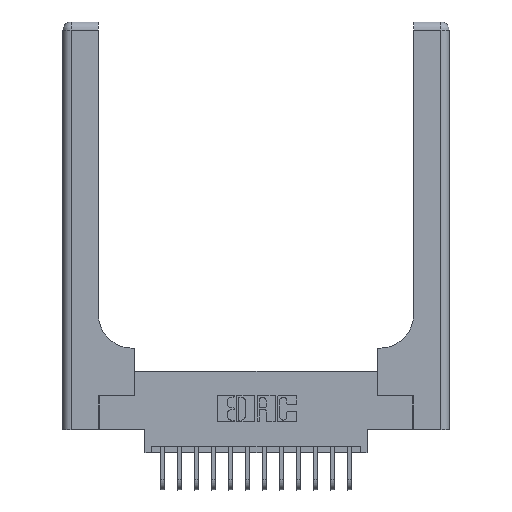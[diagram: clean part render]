
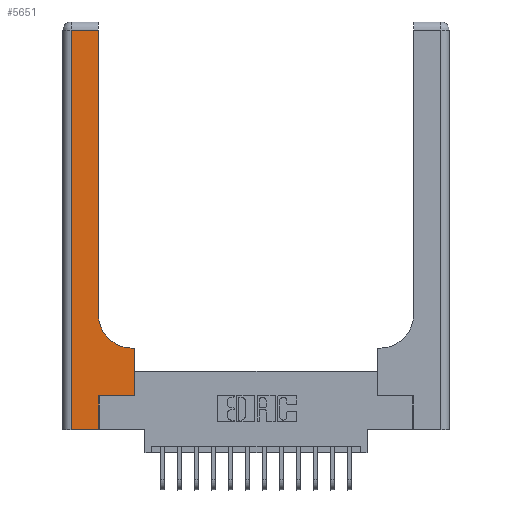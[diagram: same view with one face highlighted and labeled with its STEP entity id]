
A CAD part, top view. The second image highlights one B-rep face of the part: STEP entity #5651.
In plain terms, the highlighted planar face has unit normal (0, 0, 1).
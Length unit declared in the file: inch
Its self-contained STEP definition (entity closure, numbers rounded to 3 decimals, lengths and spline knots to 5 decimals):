
#55 = DIRECTION ( 'NONE',  ( 0., 1., 0. ) ) ;
#340 = EDGE_CURVE ( 'NONE', #1381, #548, #7350, .T. ) ;
#395 = FACE_OUTER_BOUND ( 'NONE', #15063, .T. ) ;
#422 = VERTEX_POINT ( 'NONE', #14021 ) ;
#503 = CARTESIAN_POINT ( 'NONE',  ( 0.528, 0.25, 0.37 ) ) ;
#518 = DIRECTION ( 'NONE',  ( 0., 0., -1. ) ) ;
#548 = VERTEX_POINT ( 'NONE', #11498 ) ;
#1215 = VECTOR ( 'NONE', #4240, 39.37008 ) ;
#1381 = VERTEX_POINT ( 'NONE', #14189 ) ;
#1453 = LINE ( 'NONE', #6443, #2290 ) ;
#1654 = ORIENTED_EDGE ( 'NONE', *, *, #1774, .T. ) ;
#1774 = EDGE_CURVE ( 'NONE', #3739, #4242, #1453, .T. ) ;
#1824 = DIRECTION ( 'NONE',  ( 0., 1., 0. ) ) ;
#2117 = LINE ( 'NONE', #503, #8754 ) ;
#2120 = ORIENTED_EDGE ( 'NONE', *, *, #7879, .T. ) ;
#2214 = LINE ( 'NONE', #14108, #15675 ) ;
#2290 = VECTOR ( 'NONE', #13499, 39.37008 ) ;
#2373 = LINE ( 'NONE', #11804, #15837 ) ;
#2389 = DIRECTION ( 'NONE',  ( 0., 1., 0. ) ) ;
#2402 = ORIENTED_EDGE ( 'NONE', *, *, #3684, .T. ) ;
#2925 = CARTESIAN_POINT ( 'NONE',  ( 0.528, 0.25, 0.37 ) ) ;
#3399 = VECTOR ( 'NONE', #15472, 39.37008 ) ;
#3684 = EDGE_CURVE ( 'NONE', #4242, #1381, #2117, .T. ) ;
#3739 = VERTEX_POINT ( 'NONE', #5965 ) ;
#4028 = CARTESIAN_POINT ( 'NONE',  ( 0.06, 2.94, 0.37 ) ) ;
#4240 = DIRECTION ( 'NONE',  ( 1., 0., 0. ) ) ;
#4242 = VERTEX_POINT ( 'NONE', #2925 ) ;
#4299 = CIRCLE ( 'NONE', #7024, 0.25 ) ;
#4398 = LINE ( 'NONE', #12008, #1215 ) ;
#4882 = CARTESIAN_POINT ( 'NONE',  ( 0.51, 0.85, 0.37 ) ) ;
#4971 = VERTEX_POINT ( 'NONE', #9056 ) ;
#5651 = ADVANCED_FACE ( 'NONE', ( #395 ), #12270, .F. ) ;
#5926 = VERTEX_POINT ( 'NONE', #7805 ) ;
#5965 = CARTESIAN_POINT ( 'NONE',  ( 0.265, 0.25, 0.37 ) ) ;
#6222 = DIRECTION ( 'NONE',  ( 1., 0., 0. ) ) ;
#6296 = ORIENTED_EDGE ( 'NONE', *, *, #10732, .T. ) ;
#6400 = VECTOR ( 'NONE', #8254, 39.37008 ) ;
#6443 = CARTESIAN_POINT ( 'NONE',  ( 0.265, 0.25, 0.37 ) ) ;
#6940 = CARTESIAN_POINT ( 'NONE',  ( 0., 2.94, 0.37 ) ) ;
#7024 = AXIS2_PLACEMENT_3D ( 'NONE', #4882, #13938, #6222 ) ;
#7350 = LINE ( 'NONE', #16015, #3399 ) ;
#7425 = ORIENTED_EDGE ( 'NONE', *, *, #11349, .T. ) ;
#7805 = CARTESIAN_POINT ( 'NONE',  ( 0.26, 0.85, 0.37 ) ) ;
#7879 = EDGE_CURVE ( 'NONE', #548, #5926, #4299, .T. ) ;
#8254 = DIRECTION ( 'NONE',  ( -1., 0., 0. ) ) ;
#8291 = CARTESIAN_POINT ( 'NONE',  ( 0.265, 0., 0.37 ) ) ;
#8470 = CARTESIAN_POINT ( 'NONE',  ( 0., 3., 0.37 ) ) ;
#8754 = VECTOR ( 'NONE', #1824, 39.37008 ) ;
#8766 = EDGE_CURVE ( 'NONE', #13071, #422, #10026, .T. ) ;
#9056 = CARTESIAN_POINT ( 'NONE',  ( 0.26, 2.94, 0.37 ) ) ;
#9779 = DIRECTION ( 'NONE',  ( -1., 0., 0. ) ) ;
#9852 = LINE ( 'NONE', #6940, #6400 ) ;
#10026 = LINE ( 'NONE', #14906, #12209 ) ;
#10732 = EDGE_CURVE ( 'NONE', #13164, #3739, #2214, .T. ) ;
#10830 = ORIENTED_EDGE ( 'NONE', *, *, #15857, .T. ) ;
#11349 = EDGE_CURVE ( 'NONE', #4971, #13071, #9852, .T. ) ;
#11498 = CARTESIAN_POINT ( 'NONE',  ( 0.51, 0.6, 0.37 ) ) ;
#11804 = CARTESIAN_POINT ( 'NONE',  ( 0.26, 3., 0.37 ) ) ;
#11869 = EDGE_CURVE ( 'NONE', #5926, #4971, #2373, .T. ) ;
#12008 = CARTESIAN_POINT ( 'NONE',  ( 0., 0., 0.37 ) ) ;
#12209 = VECTOR ( 'NONE', #16204, 39.37008 ) ;
#12270 = PLANE ( 'NONE',  #13577 ) ;
#13071 = VERTEX_POINT ( 'NONE', #4028 ) ;
#13164 = VERTEX_POINT ( 'NONE', #8291 ) ;
#13499 = DIRECTION ( 'NONE',  ( 1., 0., 0. ) ) ;
#13577 = AXIS2_PLACEMENT_3D ( 'NONE', #8470, #518, #9779 ) ;
#13938 = DIRECTION ( 'NONE',  ( 0., 0., -1. ) ) ;
#14021 = CARTESIAN_POINT ( 'NONE',  ( 0.06, 0., 0.37 ) ) ;
#14108 = CARTESIAN_POINT ( 'NONE',  ( 0.265, 0., 0.37 ) ) ;
#14189 = CARTESIAN_POINT ( 'NONE',  ( 0.528, 0.6, 0.37 ) ) ;
#14647 = ORIENTED_EDGE ( 'NONE', *, *, #11869, .T. ) ;
#14906 = CARTESIAN_POINT ( 'NONE',  ( 0.06, 3., 0.37 ) ) ;
#15063 = EDGE_LOOP ( 'NONE', ( #14647, #7425, #15755, #10830, #6296, #1654, #2402, #16491, #2120 ) ) ;
#15472 = DIRECTION ( 'NONE',  ( -1., 0., 0. ) ) ;
#15675 = VECTOR ( 'NONE', #2389, 39.37008 ) ;
#15755 = ORIENTED_EDGE ( 'NONE', *, *, #8766, .T. ) ;
#15837 = VECTOR ( 'NONE', #55, 39.37008 ) ;
#15857 = EDGE_CURVE ( 'NONE', #422, #13164, #4398, .T. ) ;
#16015 = CARTESIAN_POINT ( 'NONE',  ( 0.26, 0.6, 0.37 ) ) ;
#16204 = DIRECTION ( 'NONE',  ( 0., -1., 0. ) ) ;
#16491 = ORIENTED_EDGE ( 'NONE', *, *, #340, .T. ) ;
